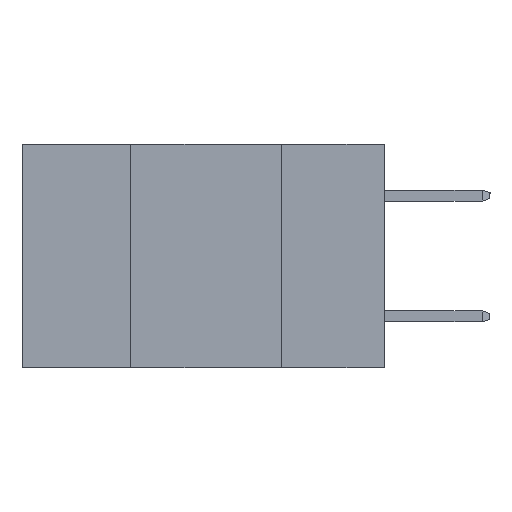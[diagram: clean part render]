
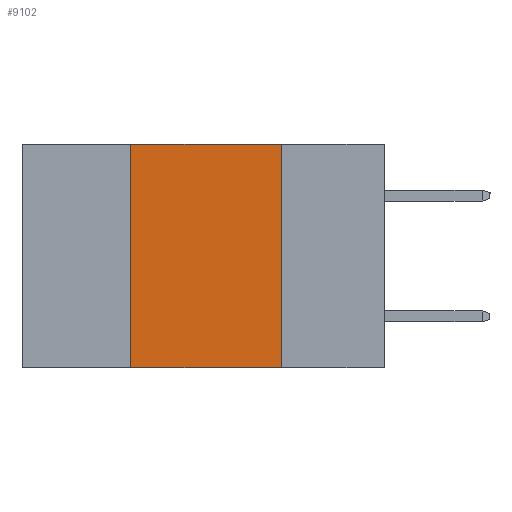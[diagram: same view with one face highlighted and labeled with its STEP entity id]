
A CAD part, left-side view. The second image highlights one B-rep face of the part: STEP entity #9102.
In plain terms, the highlighted planar face has unit normal (-1, 0, 0).
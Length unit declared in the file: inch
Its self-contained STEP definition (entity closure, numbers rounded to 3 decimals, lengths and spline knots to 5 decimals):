
#50 = DIRECTION ( 'NONE',  ( 0., -1., 0. ) ) ;
#62 = ORIENTED_EDGE ( 'NONE', *, *, #4063, .T. ) ;
#764 = CARTESIAN_POINT ( 'NONE',  ( 0., 0.42, 0. ) ) ;
#878 = DIRECTION ( 'NONE',  ( 0., 0., 1. ) ) ;
#2492 = EDGE_CURVE ( 'NONE', #3917, #7986, #7738, .T. ) ;
#2543 = CARTESIAN_POINT ( 'NONE',  ( 0., 0.42, -0.37 ) ) ;
#2681 = CARTESIAN_POINT ( 'NONE',  ( 0., 0.42, -0.37 ) ) ;
#2799 = ORIENTED_EDGE ( 'NONE', *, *, #6322, .F. ) ;
#2989 = AXIS2_PLACEMENT_3D ( 'NONE', #10756, #9894, #3154 ) ;
#3154 = DIRECTION ( 'NONE',  ( 0., 0., -1. ) ) ;
#3603 = EDGE_LOOP ( 'NONE', ( #2799, #7336, #10255, #62 ) ) ;
#3917 = VERTEX_POINT ( 'NONE', #764 ) ;
#4061 = VECTOR ( 'NONE', #878, 39.37008 ) ;
#4063 = EDGE_CURVE ( 'NONE', #4584, #7563, #7850, .T. ) ;
#4280 = CARTESIAN_POINT ( 'NONE',  ( 0., 0.6, 0. ) ) ;
#4584 = VERTEX_POINT ( 'NONE', #2681 ) ;
#4737 = VECTOR ( 'NONE', #5292, 39.37008 ) ;
#5292 = DIRECTION ( 'NONE',  ( 0., -1., 0. ) ) ;
#5317 = CARTESIAN_POINT ( 'NONE',  ( 0., 0.17, -0.37 ) ) ;
#5965 = CARTESIAN_POINT ( 'NONE',  ( 0., 0.6, -0.37 ) ) ;
#6019 = VECTOR ( 'NONE', #9420, 39.37008 ) ;
#6322 = EDGE_CURVE ( 'NONE', #7986, #7563, #7769, .T. ) ;
#6519 = FACE_OUTER_BOUND ( 'NONE', #3603, .T. ) ;
#7336 = ORIENTED_EDGE ( 'NONE', *, *, #2492, .F. ) ;
#7563 = VERTEX_POINT ( 'NONE', #5317 ) ;
#7605 = VECTOR ( 'NONE', #50, 39.37008 ) ;
#7738 = LINE ( 'NONE', #4280, #7605 ) ;
#7769 = LINE ( 'NONE', #8421, #6019 ) ;
#7803 = LINE ( 'NONE', #2543, #4061 ) ;
#7850 = LINE ( 'NONE', #5965, #4737 ) ;
#7986 = VERTEX_POINT ( 'NONE', #10677 ) ;
#8421 = CARTESIAN_POINT ( 'NONE',  ( 0., 0.17, -0.37 ) ) ;
#8819 = EDGE_CURVE ( 'NONE', #4584, #3917, #7803, .T. ) ;
#9102 = ADVANCED_FACE ( 'NONE', ( #6519 ), #10814, .F. ) ;
#9420 = DIRECTION ( 'NONE',  ( 0., 0., -1. ) ) ;
#9894 = DIRECTION ( 'NONE',  ( 1., 0., 0. ) ) ;
#10255 = ORIENTED_EDGE ( 'NONE', *, *, #8819, .F. ) ;
#10677 = CARTESIAN_POINT ( 'NONE',  ( 0., 0.17, 0. ) ) ;
#10756 = CARTESIAN_POINT ( 'NONE',  ( 0., 0.6, 0. ) ) ;
#10814 = PLANE ( 'NONE',  #2989 ) ;
